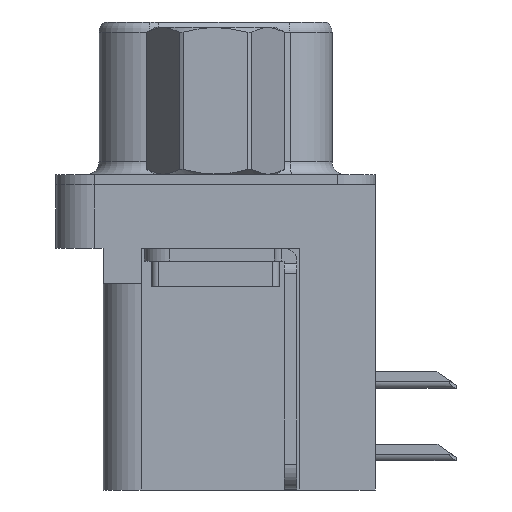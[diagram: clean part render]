
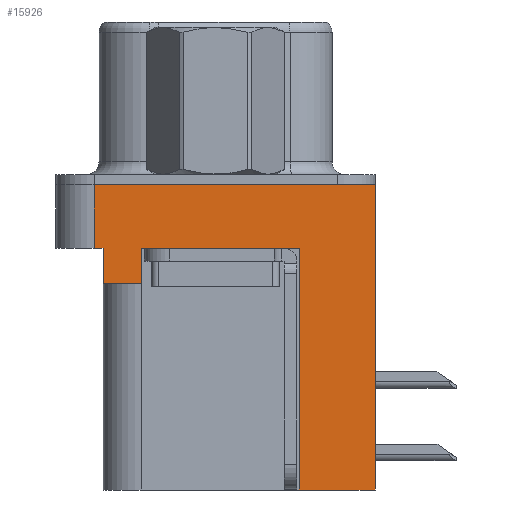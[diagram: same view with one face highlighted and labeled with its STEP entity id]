
A CAD part, left-side view. The second image highlights one B-rep face of the part: STEP entity #15926.
In plain terms, the highlighted planar face has unit normal (-1, 0, 0).
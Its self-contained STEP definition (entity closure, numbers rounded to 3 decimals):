
#11 = CARTESIAN_POINT ( 'NONE',  ( -2.935, 2.895, -3.9 ) ) ;
#91 = DIRECTION ( 'NONE',  ( 0., -1., 0. ) ) ;
#1031 = VERTEX_POINT ( 'NONE', #11 ) ;
#1055 = VERTEX_POINT ( 'NONE', #9823 ) ;
#1830 = LINE ( 'NONE', #10952, #17865 ) ;
#2671 = CARTESIAN_POINT ( 'NONE',  ( -2.935, -6.275, -12. ) ) ;
#2886 = DIRECTION ( 'NONE',  ( 0., 0., 1. ) ) ;
#2900 = DIRECTION ( 'NONE',  ( 0., -1., 0. ) ) ;
#2960 = EDGE_CURVE ( 'NONE', #21317, #10390, #22360, .T. ) ;
#3086 = ORIENTED_EDGE ( 'NONE', *, *, #8959, .T. ) ;
#3134 = DIRECTION ( 'NONE',  ( 0., -1., 0. ) ) ;
#3449 = VERTEX_POINT ( 'NONE', #13045 ) ;
#3765 = VECTOR ( 'NONE', #2886, 1000. ) ;
#4588 = CARTESIAN_POINT ( 'NONE',  ( -2.935, 2.895, -2.5 ) ) ;
#5571 = FACE_OUTER_BOUND ( 'NONE', #6091, .T. ) ;
#6053 = AXIS2_PLACEMENT_3D ( 'NONE', #16222, #7335, #9197 ) ;
#6091 = EDGE_LOOP ( 'NONE', ( #19626, #21316, #3086, #21532, #22242, #20091, #8267, #18502, #12629, #12486 ) ) ;
#6250 = DIRECTION ( 'NONE',  ( 0., 1., 0. ) ) ;
#6731 = VERTEX_POINT ( 'NONE', #11844 ) ;
#7335 = DIRECTION ( 'NONE',  ( -1., 0., 0. ) ) ;
#7362 = VECTOR ( 'NONE', #3134, 1000. ) ;
#7515 = EDGE_CURVE ( 'NONE', #8958, #6731, #15176, .T. ) ;
#7584 = VECTOR ( 'NONE', #6250, 1000. ) ;
#8085 = EDGE_CURVE ( 'NONE', #3449, #10491, #22307, .T. ) ;
#8238 = VECTOR ( 'NONE', #2900, 1000. ) ;
#8245 = EDGE_CURVE ( 'NONE', #21317, #1055, #18563, .T. ) ;
#8267 = ORIENTED_EDGE ( 'NONE', *, *, #7515, .T. ) ;
#8599 = CARTESIAN_POINT ( 'NONE',  ( -2.935, -6.275, -2.5 ) ) ;
#8768 = EDGE_CURVE ( 'NONE', #16204, #10390, #15943, .T. ) ;
#8901 = CARTESIAN_POINT ( 'NONE',  ( -2.935, 4.775, -2.5 ) ) ;
#8958 = VERTEX_POINT ( 'NONE', #4588 ) ;
#8959 = EDGE_CURVE ( 'NONE', #18856, #10491, #21658, .T. ) ;
#9197 = DIRECTION ( 'NONE',  ( 0., 0., 1. ) ) ;
#9823 = CARTESIAN_POINT ( 'NONE',  ( -2.935, -3.295, -12. ) ) ;
#10390 = VERTEX_POINT ( 'NONE', #22452 ) ;
#10466 = CARTESIAN_POINT ( 'NONE',  ( -2.935, -3.295, -12. ) ) ;
#10491 = VERTEX_POINT ( 'NONE', #18684 ) ;
#10952 = CARTESIAN_POINT ( 'NONE',  ( -2.935, 2.895, -3.9 ) ) ;
#11431 = VECTOR ( 'NONE', #23654, 1000. ) ;
#11844 = CARTESIAN_POINT ( 'NONE',  ( -2.935, -3.295, -2.5 ) ) ;
#12009 = EDGE_CURVE ( 'NONE', #1055, #6731, #16071, .T. ) ;
#12486 = ORIENTED_EDGE ( 'NONE', *, *, #2960, .T. ) ;
#12629 = ORIENTED_EDGE ( 'NONE', *, *, #8245, .F. ) ;
#12871 = CARTESIAN_POINT ( 'NONE',  ( -2.935, -6.275, -2.5 ) ) ;
#13045 = CARTESIAN_POINT ( 'NONE',  ( -2.935, 4.425, -3.9 ) ) ;
#13264 = EDGE_CURVE ( 'NONE', #18856, #16204, #23164, .T. ) ;
#13760 = VECTOR ( 'NONE', #19326, 1000. ) ;
#15176 = LINE ( 'NONE', #12871, #16295 ) ;
#15587 = CARTESIAN_POINT ( 'NONE',  ( -2.935, 4.425, -3.9 ) ) ;
#15926 = ADVANCED_FACE ( 'NONE', ( #5571 ), #18271, .T. ) ;
#15943 = LINE ( 'NONE', #21354, #7362 ) ;
#16071 = LINE ( 'NONE', #16568, #17790 ) ;
#16204 = VERTEX_POINT ( 'NONE', #19438 ) ;
#16222 = CARTESIAN_POINT ( 'NONE',  ( -2.935, -6.275, -2.5 ) ) ;
#16295 = VECTOR ( 'NONE', #91, 1000. ) ;
#16491 = DIRECTION ( 'NONE',  ( 0., 0., 1. ) ) ;
#16568 = CARTESIAN_POINT ( 'NONE',  ( -2.935, -3.295, -12. ) ) ;
#16596 = DIRECTION ( 'NONE',  ( 0., 0., 1. ) ) ;
#17163 = CARTESIAN_POINT ( 'NONE',  ( -2.935, 4.425, -3.9 ) ) ;
#17275 = LINE ( 'NONE', #17163, #7584 ) ;
#17407 = VECTOR ( 'NONE', #18927, 1000. ) ;
#17790 = VECTOR ( 'NONE', #16491, 1000. ) ;
#17865 = VECTOR ( 'NONE', #16596, 1000. ) ;
#18271 = PLANE ( 'NONE',  #6053 ) ;
#18502 = ORIENTED_EDGE ( 'NONE', *, *, #12009, .F. ) ;
#18563 = LINE ( 'NONE', #10466, #13760 ) ;
#18684 = CARTESIAN_POINT ( 'NONE',  ( -2.935, 4.425, -2.5 ) ) ;
#18856 = VERTEX_POINT ( 'NONE', #19287 ) ;
#18927 = DIRECTION ( 'NONE',  ( 0., 0., 1. ) ) ;
#19287 = CARTESIAN_POINT ( 'NONE',  ( -2.935, 4.775, -2.5 ) ) ;
#19326 = DIRECTION ( 'NONE',  ( 0., 1., 0. ) ) ;
#19372 = EDGE_CURVE ( 'NONE', #1031, #3449, #17275, .T. ) ;
#19438 = CARTESIAN_POINT ( 'NONE',  ( -2.935, 4.775, 0. ) ) ;
#19626 = ORIENTED_EDGE ( 'NONE', *, *, #8768, .F. ) ;
#20091 = ORIENTED_EDGE ( 'NONE', *, *, #23274, .T. ) ;
#21122 = CARTESIAN_POINT ( 'NONE',  ( -2.935, -6.275, -2.5 ) ) ;
#21316 = ORIENTED_EDGE ( 'NONE', *, *, #13264, .F. ) ;
#21317 = VERTEX_POINT ( 'NONE', #2671 ) ;
#21354 = CARTESIAN_POINT ( 'NONE',  ( -2.935, -6.275, 0. ) ) ;
#21532 = ORIENTED_EDGE ( 'NONE', *, *, #8085, .F. ) ;
#21658 = LINE ( 'NONE', #21122, #8238 ) ;
#22242 = ORIENTED_EDGE ( 'NONE', *, *, #19372, .F. ) ;
#22307 = LINE ( 'NONE', #15587, #17407 ) ;
#22360 = LINE ( 'NONE', #8599, #3765 ) ;
#22452 = CARTESIAN_POINT ( 'NONE',  ( -2.935, -6.275, 0. ) ) ;
#23164 = LINE ( 'NONE', #8901, #11431 ) ;
#23274 = EDGE_CURVE ( 'NONE', #1031, #8958, #1830, .T. ) ;
#23654 = DIRECTION ( 'NONE',  ( 0., 0., 1. ) ) ;
